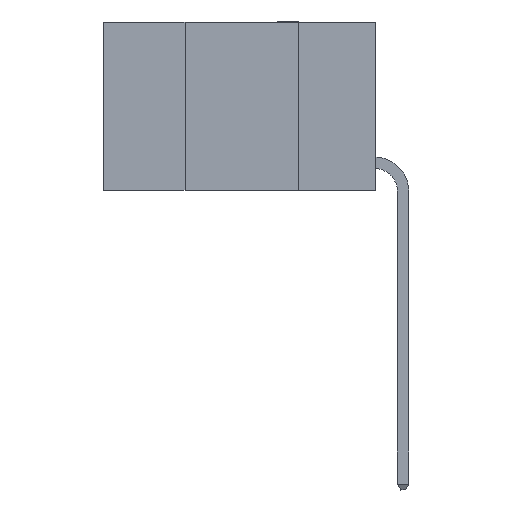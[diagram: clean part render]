
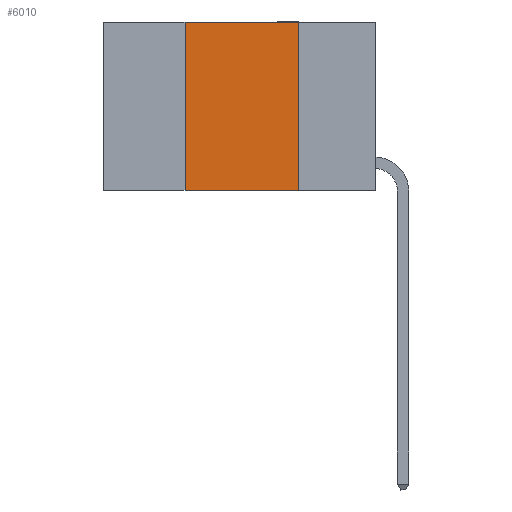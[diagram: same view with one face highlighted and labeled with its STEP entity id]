
A CAD part, left-side view. The second image highlights one B-rep face of the part: STEP entity #6010.
In plain terms, the highlighted planar face has unit normal (-1, 0, 0).
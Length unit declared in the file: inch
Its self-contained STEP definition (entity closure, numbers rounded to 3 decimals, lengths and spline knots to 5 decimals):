
#349 = AXIS2_PLACEMENT_3D ( 'NONE', #4619, #2854, #3737 ) ;
#570 = VERTEX_POINT ( 'NONE', #11206 ) ;
#642 = VERTEX_POINT ( 'NONE', #3885 ) ;
#787 = ORIENTED_EDGE ( 'NONE', *, *, #7761, .F. ) ;
#1023 = PLANE ( 'NONE',  #349 ) ;
#1075 = VECTOR ( 'NONE', #4105, 39.37008 ) ;
#1580 = VERTEX_POINT ( 'NONE', #8401 ) ;
#2854 = DIRECTION ( 'NONE',  ( 1., 0., 0. ) ) ;
#3535 = CARTESIAN_POINT ( 'NONE',  ( 0., 0.17, 0. ) ) ;
#3737 = DIRECTION ( 'NONE',  ( 0., 0., -1. ) ) ;
#3849 = FACE_OUTER_BOUND ( 'NONE', #7869, .T. ) ;
#3885 = CARTESIAN_POINT ( 'NONE',  ( 0., 0.42, 0. ) ) ;
#4105 = DIRECTION ( 'NONE',  ( 0., -1., 0. ) ) ;
#4273 = LINE ( 'NONE', #11233, #6756 ) ;
#4553 = ORIENTED_EDGE ( 'NONE', *, *, #7822, .F. ) ;
#4619 = CARTESIAN_POINT ( 'NONE',  ( 0., 0.6, 0. ) ) ;
#5652 = EDGE_CURVE ( 'NONE', #570, #11412, #9483, .T. ) ;
#5806 = DIRECTION ( 'NONE',  ( 0., 0., 1. ) ) ;
#6010 = ADVANCED_FACE ( 'NONE', ( #3849 ), #1023, .F. ) ;
#6756 = VECTOR ( 'NONE', #5806, 39.37008 ) ;
#6941 = CARTESIAN_POINT ( 'NONE',  ( 0., 0.17, -0.37 ) ) ;
#7145 = DIRECTION ( 'NONE',  ( 0., 0., -1. ) ) ;
#7424 = EDGE_CURVE ( 'NONE', #570, #642, #4273, .T. ) ;
#7563 = DIRECTION ( 'NONE',  ( 0., -1., 0. ) ) ;
#7761 = EDGE_CURVE ( 'NONE', #1580, #11412, #11678, .T. ) ;
#7822 = EDGE_CURVE ( 'NONE', #642, #1580, #8534, .T. ) ;
#7869 = EDGE_LOOP ( 'NONE', ( #787, #4553, #9556, #11692 ) ) ;
#7937 = VECTOR ( 'NONE', #7145, 39.37008 ) ;
#8401 = CARTESIAN_POINT ( 'NONE',  ( 0., 0.17, 0. ) ) ;
#8534 = LINE ( 'NONE', #10302, #8876 ) ;
#8876 = VECTOR ( 'NONE', #7563, 39.37008 ) ;
#9483 = LINE ( 'NONE', #9546, #1075 ) ;
#9546 = CARTESIAN_POINT ( 'NONE',  ( 0., 0.6, -0.37 ) ) ;
#9556 = ORIENTED_EDGE ( 'NONE', *, *, #7424, .F. ) ;
#10302 = CARTESIAN_POINT ( 'NONE',  ( 0., 0.6, 0. ) ) ;
#11206 = CARTESIAN_POINT ( 'NONE',  ( 0., 0.42, -0.37 ) ) ;
#11233 = CARTESIAN_POINT ( 'NONE',  ( 0., 0.42, 0. ) ) ;
#11412 = VERTEX_POINT ( 'NONE', #6941 ) ;
#11678 = LINE ( 'NONE', #3535, #7937 ) ;
#11692 = ORIENTED_EDGE ( 'NONE', *, *, #5652, .T. ) ;
